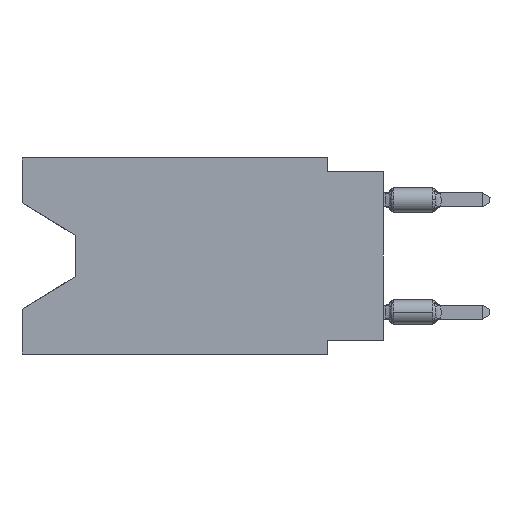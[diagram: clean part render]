
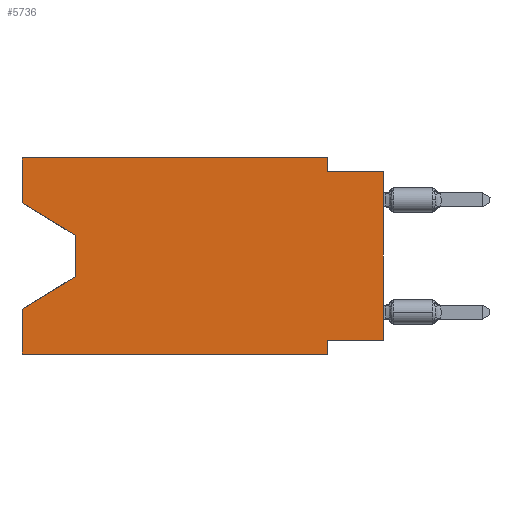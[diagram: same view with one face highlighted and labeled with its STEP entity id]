
A CAD part, left-side view. The second image highlights one B-rep face of the part: STEP entity #5736.
In plain terms, the highlighted planar face has unit normal (-1, 0, 0).
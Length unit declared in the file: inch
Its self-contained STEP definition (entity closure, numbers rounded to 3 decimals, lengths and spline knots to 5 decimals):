
#764 = VERTEX_POINT ( 'NONE', #8812 ) ;
#1812 = EDGE_LOOP ( 'NONE', ( #29306, #9127, #15817, #33002, #39607, #40756, #25260, #15690, #24910, #5211, #30231, #40566 ) ) ;
#3126 = EDGE_CURVE ( 'NONE', #5725, #20617, #28615, .T. ) ;
#3990 = DIRECTION ( 'NONE',  ( 1., 0., 0. ) ) ;
#4211 = CARTESIAN_POINT ( 'NONE',  ( 0., 0.55, -0.138 ) ) ;
#4775 = CARTESIAN_POINT ( 'NONE',  ( 0., 0.645, -0.35 ) ) ;
#5170 = VERTEX_POINT ( 'NONE', #12435 ) ;
#5211 = ORIENTED_EDGE ( 'NONE', *, *, #14191, .F. ) ;
#5446 = VECTOR ( 'NONE', #30546, 39.37008 ) ;
#5620 = EDGE_CURVE ( 'NONE', #20617, #28883, #22692, .T. ) ;
#5725 = VERTEX_POINT ( 'NONE', #4211 ) ;
#5736 = ADVANCED_FACE ( 'NONE', ( #37020 ), #36795, .F. ) ;
#6234 = VERTEX_POINT ( 'NONE', #8404 ) ;
#7190 = VECTOR ( 'NONE', #14266, 39.37008 ) ;
#7438 = CARTESIAN_POINT ( 'NONE',  ( 0., 0.645, 0. ) ) ;
#7968 = LINE ( 'NONE', #33910, #20028 ) ;
#8404 = CARTESIAN_POINT ( 'NONE',  ( 0., 0.645, -0.35 ) ) ;
#8812 = CARTESIAN_POINT ( 'NONE',  ( 0., 0.645, -0.08025 ) ) ;
#9127 = ORIENTED_EDGE ( 'NONE', *, *, #3126, .T. ) ;
#9637 = DIRECTION ( 'NONE',  ( 0., 0., 1. ) ) ;
#10026 = CARTESIAN_POINT ( 'NONE',  ( 0., 0.55, -0.212 ) ) ;
#10592 = CARTESIAN_POINT ( 'NONE',  ( 0., 0.1, -0.025 ) ) ;
#10858 = VECTOR ( 'NONE', #25680, 39.37008 ) ;
#11004 = LINE ( 'NONE', #4775, #17847 ) ;
#11072 = DIRECTION ( 'NONE',  ( 0., 0., -1. ) ) ;
#11523 = EDGE_CURVE ( 'NONE', #16346, #33017, #30563, .T. ) ;
#11734 = LINE ( 'NONE', #30258, #31419 ) ;
#12080 = VECTOR ( 'NONE', #25189, 39.37008 ) ;
#12131 = DIRECTION ( 'NONE',  ( 0., 0., -1. ) ) ;
#12400 = EDGE_CURVE ( 'NONE', #41503, #28789, #11734, .T. ) ;
#12435 = CARTESIAN_POINT ( 'NONE',  ( 0., 0.645, 0. ) ) ;
#13317 = CARTESIAN_POINT ( 'NONE',  ( 0., 0., -0.025 ) ) ;
#13750 = CARTESIAN_POINT ( 'NONE',  ( 0., 0.645, -0.26975 ) ) ;
#14014 = DIRECTION ( 'NONE',  ( 0., 0., -1. ) ) ;
#14147 = EDGE_CURVE ( 'NONE', #6234, #28789, #11004, .T. ) ;
#14191 = EDGE_CURVE ( 'NONE', #30631, #16346, #30745, .T. ) ;
#14266 = DIRECTION ( 'NONE',  ( 0., 0., 1. ) ) ;
#14443 = CARTESIAN_POINT ( 'NONE',  ( 0., 0.1, 0. ) ) ;
#15690 = ORIENTED_EDGE ( 'NONE', *, *, #26504, .T. ) ;
#15817 = ORIENTED_EDGE ( 'NONE', *, *, #5620, .T. ) ;
#16092 = CARTESIAN_POINT ( 'NONE',  ( 0., 0.55, -0.212 ) ) ;
#16329 = CARTESIAN_POINT ( 'NONE',  ( 0., 0.1, -0.325 ) ) ;
#16346 = VERTEX_POINT ( 'NONE', #10592 ) ;
#16850 = CARTESIAN_POINT ( 'NONE',  ( 0., 0.645, -0.08025 ) ) ;
#17284 = LINE ( 'NONE', #33981, #7190 ) ;
#17847 = VECTOR ( 'NONE', #26681, 39.37008 ) ;
#17882 = CARTESIAN_POINT ( 'NONE',  ( 0., 0.1, 0. ) ) ;
#18108 = CARTESIAN_POINT ( 'NONE',  ( 0., 0., -0.325 ) ) ;
#18535 = VECTOR ( 'NONE', #14014, 39.37008 ) ;
#19034 = CARTESIAN_POINT ( 'NONE',  ( 0., 0.645, 0. ) ) ;
#19338 = CARTESIAN_POINT ( 'NONE',  ( 0., 0.1, -0.35 ) ) ;
#20028 = VECTOR ( 'NONE', #20836, 39.37008 ) ;
#20617 = VERTEX_POINT ( 'NONE', #16092 ) ;
#20836 = DIRECTION ( 'NONE',  ( 0., 0., 1. ) ) ;
#21089 = LINE ( 'NONE', #18108, #5446 ) ;
#21235 = EDGE_CURVE ( 'NONE', #5170, #30631, #22250, .T. ) ;
#22250 = LINE ( 'NONE', #19034, #27274 ) ;
#22335 = CARTESIAN_POINT ( 'NONE',  ( 0., 0., -0.325 ) ) ;
#22692 = LINE ( 'NONE', #10026, #10858 ) ;
#23711 = DIRECTION ( 'NONE',  ( 0., -0.855, -0.519 ) ) ;
#24910 = ORIENTED_EDGE ( 'NONE', *, *, #11523, .F. ) ;
#24990 = EDGE_CURVE ( 'NONE', #28700, #41503, #21089, .T. ) ;
#25189 = DIRECTION ( 'NONE',  ( 0., 0., -1. ) ) ;
#25260 = ORIENTED_EDGE ( 'NONE', *, *, #24990, .F. ) ;
#25402 = CARTESIAN_POINT ( 'NONE',  ( 0., 0.55, -0.138 ) ) ;
#25680 = DIRECTION ( 'NONE',  ( 0., 0.855, -0.519 ) ) ;
#25932 = LINE ( 'NONE', #39018, #38600 ) ;
#26504 = EDGE_CURVE ( 'NONE', #28700, #33017, #7968, .T. ) ;
#26681 = DIRECTION ( 'NONE',  ( 0., -1., 0. ) ) ;
#27274 = VECTOR ( 'NONE', #30170, 39.37008 ) ;
#28294 = EDGE_CURVE ( 'NONE', #6234, #28883, #25932, .T. ) ;
#28615 = LINE ( 'NONE', #25402, #12080 ) ;
#28700 = VERTEX_POINT ( 'NONE', #22335 ) ;
#28789 = VERTEX_POINT ( 'NONE', #19338 ) ;
#28883 = VERTEX_POINT ( 'NONE', #13750 ) ;
#29306 = ORIENTED_EDGE ( 'NONE', *, *, #29741, .T. ) ;
#29741 = EDGE_CURVE ( 'NONE', #764, #5725, #36154, .T. ) ;
#29881 = EDGE_CURVE ( 'NONE', #764, #5170, #17284, .T. ) ;
#30039 = AXIS2_PLACEMENT_3D ( 'NONE', #7438, #3990, #11072 ) ;
#30170 = DIRECTION ( 'NONE',  ( 0., -1., 0. ) ) ;
#30231 = ORIENTED_EDGE ( 'NONE', *, *, #21235, .F. ) ;
#30258 = CARTESIAN_POINT ( 'NONE',  ( 0., 0.1, -0.35 ) ) ;
#30546 = DIRECTION ( 'NONE',  ( 0., 1., 0. ) ) ;
#30563 = LINE ( 'NONE', #34407, #40570 ) ;
#30631 = VERTEX_POINT ( 'NONE', #14443 ) ;
#30745 = LINE ( 'NONE', #17882, #18535 ) ;
#31419 = VECTOR ( 'NONE', #12131, 39.37008 ) ;
#33002 = ORIENTED_EDGE ( 'NONE', *, *, #28294, .F. ) ;
#33017 = VERTEX_POINT ( 'NONE', #13317 ) ;
#33910 = CARTESIAN_POINT ( 'NONE',  ( 0., 0., 0. ) ) ;
#33981 = CARTESIAN_POINT ( 'NONE',  ( 0., 0.645, 0. ) ) ;
#34407 = CARTESIAN_POINT ( 'NONE',  ( 0., 0., -0.025 ) ) ;
#36154 = LINE ( 'NONE', #16850, #42109 ) ;
#36795 = PLANE ( 'NONE',  #30039 ) ;
#37020 = FACE_OUTER_BOUND ( 'NONE', #1812, .T. ) ;
#38600 = VECTOR ( 'NONE', #9637, 39.37008 ) ;
#39018 = CARTESIAN_POINT ( 'NONE',  ( 0., 0.645, 0. ) ) ;
#39607 = ORIENTED_EDGE ( 'NONE', *, *, #14147, .T. ) ;
#40566 = ORIENTED_EDGE ( 'NONE', *, *, #29881, .F. ) ;
#40570 = VECTOR ( 'NONE', #41052, 39.37008 ) ;
#40756 = ORIENTED_EDGE ( 'NONE', *, *, #12400, .F. ) ;
#41052 = DIRECTION ( 'NONE',  ( 0., -1., 0. ) ) ;
#41503 = VERTEX_POINT ( 'NONE', #16329 ) ;
#42109 = VECTOR ( 'NONE', #23711, 39.37008 ) ;
